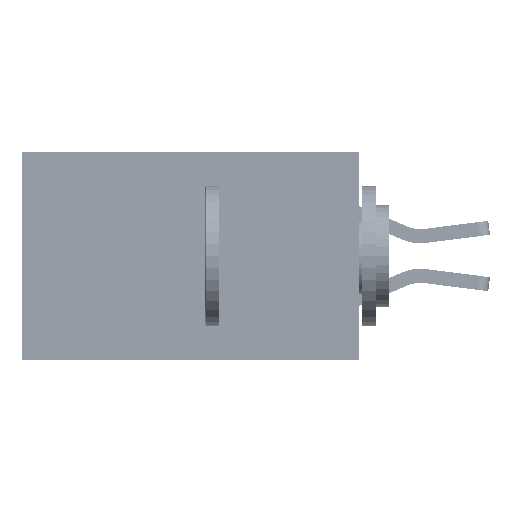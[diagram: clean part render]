
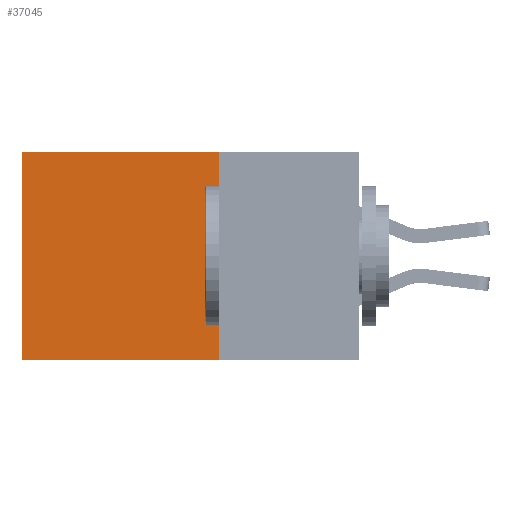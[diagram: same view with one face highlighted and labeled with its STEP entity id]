
A CAD part, left-side view. The second image highlights one B-rep face of the part: STEP entity #37045.
In plain terms, the highlighted planar face has unit normal (-1, 0, 0).
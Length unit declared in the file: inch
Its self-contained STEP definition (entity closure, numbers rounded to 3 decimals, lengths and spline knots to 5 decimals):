
#2670 = ORIENTED_EDGE ( 'NONE', *, *, #24659, .F. ) ;
#5851 = ORIENTED_EDGE ( 'NONE', *, *, #41511, .T. ) ;
#6672 = VECTOR ( 'NONE', #14732, 39.37008 ) ;
#7212 = CARTESIAN_POINT ( 'NONE',  ( 0.2875, 0.25, 0. ) ) ;
#8406 = EDGE_CURVE ( 'NONE', #25442, #16107, #32701, .T. ) ;
#12373 = CARTESIAN_POINT ( 'NONE',  ( 0.2875, 0.25, 0. ) ) ;
#14732 = DIRECTION ( 'NONE',  ( 0., 1., 0. ) ) ;
#16107 = VERTEX_POINT ( 'NONE', #26066 ) ;
#16344 = DIRECTION ( 'NONE',  ( 0., 0., -1. ) ) ;
#17540 = CARTESIAN_POINT ( 'NONE',  ( 0.2875, 0.6, -0.37 ) ) ;
#17870 = VERTEX_POINT ( 'NONE', #17540 ) ;
#18636 = DIRECTION ( 'NONE',  ( 1., 0., 0. ) ) ;
#20004 = CARTESIAN_POINT ( 'NONE',  ( 0.2875, 0.25, -0.37 ) ) ;
#20196 = AXIS2_PLACEMENT_3D ( 'NONE', #38178, #18636, #42426 ) ;
#23591 = FACE_OUTER_BOUND ( 'NONE', #35858, .T. ) ;
#23636 = VERTEX_POINT ( 'NONE', #46430 ) ;
#24381 = DIRECTION ( 'NONE',  ( 0., 0., -1. ) ) ;
#24528 = LINE ( 'NONE', #49712, #6672 ) ;
#24659 = EDGE_CURVE ( 'NONE', #16107, #17870, #33308, .T. ) ;
#25442 = VERTEX_POINT ( 'NONE', #7212 ) ;
#26066 = CARTESIAN_POINT ( 'NONE',  ( 0.2875, 0.25, -0.37 ) ) ;
#29618 = VECTOR ( 'NONE', #24381, 39.37008 ) ;
#30258 = PLANE ( 'NONE',  #20196 ) ;
#32701 = LINE ( 'NONE', #12373, #29618 ) ;
#33308 = LINE ( 'NONE', #20004, #40661 ) ;
#33333 = VECTOR ( 'NONE', #16344, 39.37008 ) ;
#35858 = EDGE_LOOP ( 'NONE', ( #46355, #2670, #44316, #5851 ) ) ;
#37045 = ADVANCED_FACE ( 'NONE', ( #23591 ), #30258, .F. ) ;
#38178 = CARTESIAN_POINT ( 'NONE',  ( 0.2875, 0.25, 0. ) ) ;
#39633 = CARTESIAN_POINT ( 'NONE',  ( 0.2875, 0.6, 0. ) ) ;
#40661 = VECTOR ( 'NONE', #47409, 39.37008 ) ;
#41511 = EDGE_CURVE ( 'NONE', #25442, #23636, #24528, .T. ) ;
#42426 = DIRECTION ( 'NONE',  ( 0., 0., -1. ) ) ;
#43718 = LINE ( 'NONE', #39633, #33333 ) ;
#44316 = ORIENTED_EDGE ( 'NONE', *, *, #8406, .F. ) ;
#46355 = ORIENTED_EDGE ( 'NONE', *, *, #50328, .T. ) ;
#46430 = CARTESIAN_POINT ( 'NONE',  ( 0.2875, 0.6, 0. ) ) ;
#47409 = DIRECTION ( 'NONE',  ( 0., 1., 0. ) ) ;
#49712 = CARTESIAN_POINT ( 'NONE',  ( 0.2875, 0.25, 0. ) ) ;
#50328 = EDGE_CURVE ( 'NONE', #23636, #17870, #43718, .T. ) ;
